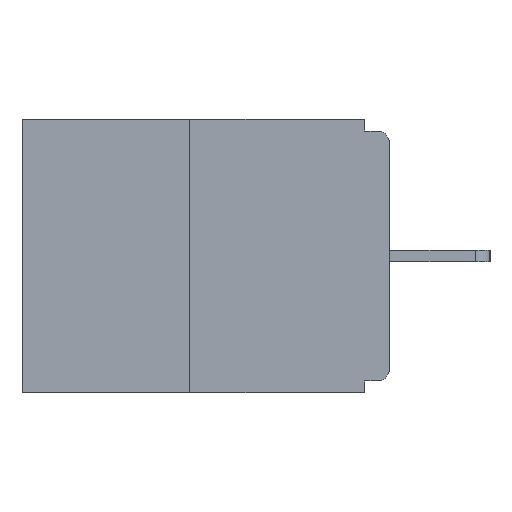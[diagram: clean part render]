
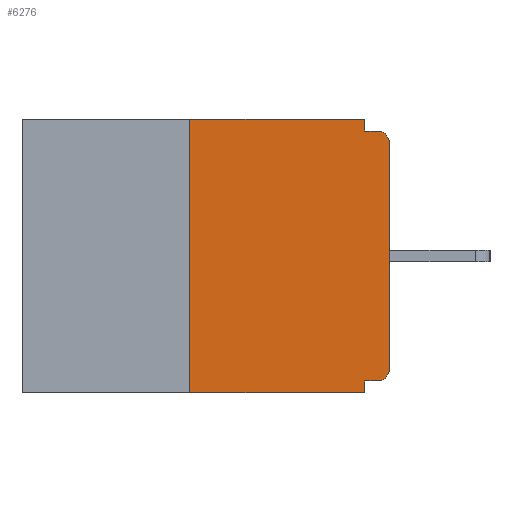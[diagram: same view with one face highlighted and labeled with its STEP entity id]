
A CAD part, left-side view. The second image highlights one B-rep face of the part: STEP entity #6276.
In plain terms, the highlighted planar face has unit normal (-1, 0, 0).
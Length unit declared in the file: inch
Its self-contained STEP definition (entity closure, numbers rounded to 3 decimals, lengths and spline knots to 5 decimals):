
#42 = EDGE_CURVE ( 'NONE', #3235, #7598, #2804, .T. ) ;
#138 = VERTEX_POINT ( 'NONE', #5569 ) ;
#193 = CARTESIAN_POINT ( 'NONE',  ( 0., 0.015, -0.015 ) ) ;
#278 = CARTESIAN_POINT ( 'NONE',  ( 0., 0., -0.328 ) ) ;
#313 = AXIS2_PLACEMENT_3D ( 'NONE', #7717, #16497, #8998 ) ;
#529 = VERTEX_POINT ( 'NONE', #10830 ) ;
#561 = CARTESIAN_POINT ( 'NONE',  ( 0., 0.031, -0.015 ) ) ;
#877 = ORIENTED_EDGE ( 'NONE', *, *, #9195, .T. ) ;
#940 = CARTESIAN_POINT ( 'NONE',  ( 0., 0.25, 0. ) ) ;
#1006 = DIRECTION ( 'NONE',  ( 0., 0., 1. ) ) ;
#1341 = EDGE_CURVE ( 'NONE', #10066, #6309, #13419, .T. ) ;
#1576 = FACE_OUTER_BOUND ( 'NONE', #4022, .T. ) ;
#1628 = VECTOR ( 'NONE', #12288, 39.37008 ) ;
#1745 = DIRECTION ( 'NONE',  ( 0., -1., 0. ) ) ;
#1804 = CARTESIAN_POINT ( 'NONE',  ( 0., 0., -0.015 ) ) ;
#2622 = CARTESIAN_POINT ( 'NONE',  ( 0., 0.46, -0.343 ) ) ;
#2686 = DIRECTION ( 'NONE',  ( 0., 0., 1. ) ) ;
#2804 = CIRCLE ( 'NONE', #10691, 0.015 ) ;
#2921 = VERTEX_POINT ( 'NONE', #561 ) ;
#2962 = VECTOR ( 'NONE', #1006, 39.37008 ) ;
#3134 = CARTESIAN_POINT ( 'NONE',  ( 0., 0.031, -0.343 ) ) ;
#3212 = DIRECTION ( 'NONE',  ( 0., 1., 0. ) ) ;
#3235 = VERTEX_POINT ( 'NONE', #3986 ) ;
#3488 = EDGE_CURVE ( 'NONE', #3235, #11802, #3757, .T. ) ;
#3757 = LINE ( 'NONE', #278, #17024 ) ;
#3986 = CARTESIAN_POINT ( 'NONE',  ( 0., 0.015, -0.328 ) ) ;
#4022 = EDGE_LOOP ( 'NONE', ( #14418, #11248, #877, #8300, #14957, #12007, #9493, #12776, #9893, #13168 ) ) ;
#4099 = DIRECTION ( 'NONE',  ( 0., -1., 0. ) ) ;
#4265 = DIRECTION ( 'NONE',  ( 0., -1., 0. ) ) ;
#4385 = CARTESIAN_POINT ( 'NONE',  ( 0., 0., 0. ) ) ;
#4454 = EDGE_CURVE ( 'NONE', #7598, #138, #11163, .T. ) ;
#5045 = EDGE_CURVE ( 'NONE', #529, #2921, #12267, .T. ) ;
#5328 = VECTOR ( 'NONE', #1745, 39.37008 ) ;
#5569 = CARTESIAN_POINT ( 'NONE',  ( 0., 0., -0.03 ) ) ;
#6276 = ADVANCED_FACE ( 'NONE', ( #1576 ), #15876, .F. ) ;
#6309 = VERTEX_POINT ( 'NONE', #15269 ) ;
#6532 = LINE ( 'NONE', #3134, #9161 ) ;
#7272 = EDGE_CURVE ( 'NONE', #2921, #11949, #8879, .T. ) ;
#7288 = DIRECTION ( 'NONE',  ( 0., 0., -1. ) ) ;
#7314 = LINE ( 'NONE', #14514, #16924 ) ;
#7598 = VERTEX_POINT ( 'NONE', #9117 ) ;
#7717 = CARTESIAN_POINT ( 'NONE',  ( 0., 0.015, -0.03 ) ) ;
#8300 = ORIENTED_EDGE ( 'NONE', *, *, #16701, .F. ) ;
#8879 = LINE ( 'NONE', #1804, #5328 ) ;
#8998 = DIRECTION ( 'NONE',  ( 0., 0., -1. ) ) ;
#9093 = AXIS2_PLACEMENT_3D ( 'NONE', #15829, #15776, #15760 ) ;
#9117 = CARTESIAN_POINT ( 'NONE',  ( 0., 0., -0.313 ) ) ;
#9161 = VECTOR ( 'NONE', #13597, 39.37008 ) ;
#9195 = EDGE_CURVE ( 'NONE', #10066, #16103, #10277, .T. ) ;
#9259 = CARTESIAN_POINT ( 'NONE',  ( 0., 0.015, -0.313 ) ) ;
#9493 = ORIENTED_EDGE ( 'NONE', *, *, #4454, .T. ) ;
#9630 = CARTESIAN_POINT ( 'NONE',  ( 0., 0.031, -0.328 ) ) ;
#9858 = VECTOR ( 'NONE', #4099, 39.37008 ) ;
#9893 = ORIENTED_EDGE ( 'NONE', *, *, #7272, .F. ) ;
#10066 = VERTEX_POINT ( 'NONE', #15743 ) ;
#10277 = LINE ( 'NONE', #2622, #9858 ) ;
#10334 = CIRCLE ( 'NONE', #313, 0.015 ) ;
#10691 = AXIS2_PLACEMENT_3D ( 'NONE', #9259, #12117, #7288 ) ;
#10830 = CARTESIAN_POINT ( 'NONE',  ( 0., 0.031, 0. ) ) ;
#11109 = EDGE_CURVE ( 'NONE', #6309, #529, #7314, .T. ) ;
#11163 = LINE ( 'NONE', #4385, #14872 ) ;
#11248 = ORIENTED_EDGE ( 'NONE', *, *, #1341, .F. ) ;
#11438 = EDGE_CURVE ( 'NONE', #138, #11949, #10334, .T. ) ;
#11802 = VERTEX_POINT ( 'NONE', #9630 ) ;
#11949 = VERTEX_POINT ( 'NONE', #193 ) ;
#12007 = ORIENTED_EDGE ( 'NONE', *, *, #42, .T. ) ;
#12117 = DIRECTION ( 'NONE',  ( -1., 0., 0. ) ) ;
#12267 = LINE ( 'NONE', #12695, #1628 ) ;
#12288 = DIRECTION ( 'NONE',  ( 0., 0., -1. ) ) ;
#12695 = CARTESIAN_POINT ( 'NONE',  ( 0., 0.031, 0. ) ) ;
#12776 = ORIENTED_EDGE ( 'NONE', *, *, #11438, .T. ) ;
#13168 = ORIENTED_EDGE ( 'NONE', *, *, #5045, .F. ) ;
#13419 = LINE ( 'NONE', #940, #2962 ) ;
#13597 = DIRECTION ( 'NONE',  ( 0., 0., -1. ) ) ;
#14418 = ORIENTED_EDGE ( 'NONE', *, *, #11109, .F. ) ;
#14514 = CARTESIAN_POINT ( 'NONE',  ( 0., 0.46, 0. ) ) ;
#14872 = VECTOR ( 'NONE', #2686, 39.37008 ) ;
#14957 = ORIENTED_EDGE ( 'NONE', *, *, #3488, .F. ) ;
#15011 = CARTESIAN_POINT ( 'NONE',  ( 0., 0.031, -0.343 ) ) ;
#15269 = CARTESIAN_POINT ( 'NONE',  ( 0., 0.25, 0. ) ) ;
#15743 = CARTESIAN_POINT ( 'NONE',  ( 0., 0.25, -0.343 ) ) ;
#15760 = DIRECTION ( 'NONE',  ( 0., 0., -1. ) ) ;
#15776 = DIRECTION ( 'NONE',  ( 1., 0., 0. ) ) ;
#15829 = CARTESIAN_POINT ( 'NONE',  ( 0., 0.46, 0. ) ) ;
#15876 = PLANE ( 'NONE',  #9093 ) ;
#16103 = VERTEX_POINT ( 'NONE', #15011 ) ;
#16497 = DIRECTION ( 'NONE',  ( -1., 0., 0. ) ) ;
#16701 = EDGE_CURVE ( 'NONE', #11802, #16103, #6532, .T. ) ;
#16924 = VECTOR ( 'NONE', #4265, 39.37008 ) ;
#17024 = VECTOR ( 'NONE', #3212, 39.37008 ) ;
